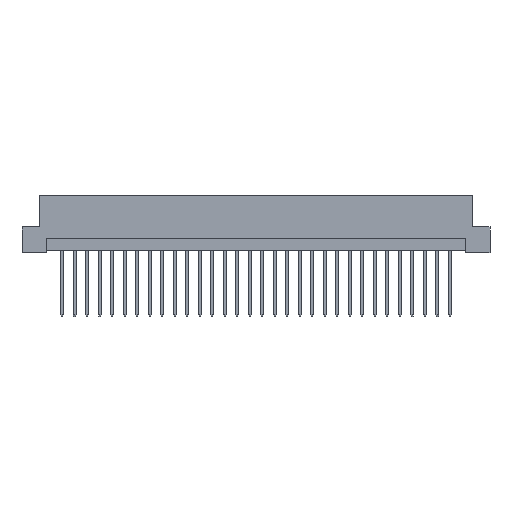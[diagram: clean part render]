
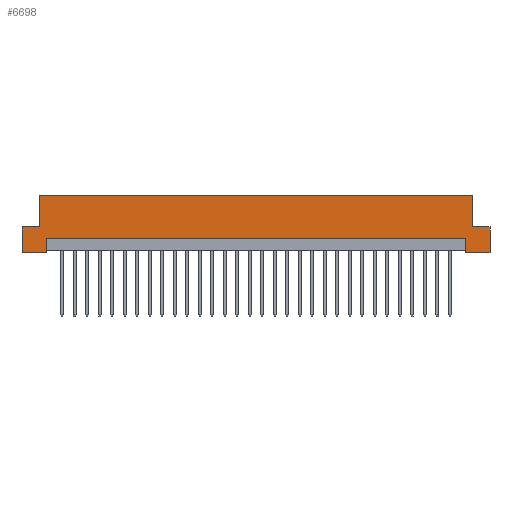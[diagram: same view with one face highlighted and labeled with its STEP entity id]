
A CAD part, front view. The second image highlights one B-rep face of the part: STEP entity #6698.
In plain terms, the highlighted planar face has unit normal (0, -1, 0).
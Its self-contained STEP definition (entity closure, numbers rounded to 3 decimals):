
#183 = VECTOR ( 'NONE', #7089, 1000. ) ;
#334 = DIRECTION ( 'NONE',  ( 1., 0., 0. ) ) ;
#344 = CARTESIAN_POINT ( 'NONE',  ( 44., 0., 11.6 ) ) ;
#518 = CARTESIAN_POINT ( 'NONE',  ( -42.6, 0., 0. ) ) ;
#773 = EDGE_CURVE ( 'NONE', #15670, #1671, #16305, .T. ) ;
#828 = LINE ( 'NONE', #3262, #14759 ) ;
#1134 = LINE ( 'NONE', #2794, #183 ) ;
#1329 = VERTEX_POINT ( 'NONE', #9438 ) ;
#1596 = VERTEX_POINT ( 'NONE', #9137 ) ;
#1671 = VERTEX_POINT ( 'NONE', #344 ) ;
#1858 = CARTESIAN_POINT ( 'NONE',  ( -42.6, 0., 0.5 ) ) ;
#1908 = VECTOR ( 'NONE', #10452, 1000. ) ;
#2086 = VERTEX_POINT ( 'NONE', #518 ) ;
#2103 = EDGE_CURVE ( 'NONE', #15670, #17255, #6191, .T. ) ;
#2208 = LINE ( 'NONE', #7899, #12714 ) ;
#2485 = VECTOR ( 'NONE', #11532, 1000. ) ;
#2656 = VECTOR ( 'NONE', #16609, 1000. ) ;
#2723 = DIRECTION ( 'NONE',  ( 0., 0., 1. ) ) ;
#2794 = CARTESIAN_POINT ( 'NONE',  ( 42.6, 0., 2.9 ) ) ;
#3262 = CARTESIAN_POINT ( 'NONE',  ( 47.5, 0., 0. ) ) ;
#3556 = VECTOR ( 'NONE', #7881, 1000. ) ;
#3605 = CARTESIAN_POINT ( 'NONE',  ( 42.6, 0., 0. ) ) ;
#3652 = VERTEX_POINT ( 'NONE', #17340 ) ;
#3809 = AXIS2_PLACEMENT_3D ( 'NONE', #18094, #5425, #2723 ) ;
#4188 = VECTOR ( 'NONE', #16476, 1000. ) ;
#4403 = CARTESIAN_POINT ( 'NONE',  ( 47.5, 0., 0. ) ) ;
#4410 = EDGE_CURVE ( 'NONE', #2086, #11112, #16179, .T. ) ;
#4904 = VERTEX_POINT ( 'NONE', #4403 ) ;
#4984 = LINE ( 'NONE', #10686, #2656 ) ;
#5258 = CARTESIAN_POINT ( 'NONE',  ( -47.5, 0., 11.6 ) ) ;
#5264 = VERTEX_POINT ( 'NONE', #6732 ) ;
#5296 = ORIENTED_EDGE ( 'NONE', *, *, #12866, .F. ) ;
#5404 = ORIENTED_EDGE ( 'NONE', *, *, #8252, .F. ) ;
#5425 = DIRECTION ( 'NONE',  ( 0., 1., 0. ) ) ;
#5496 = EDGE_CURVE ( 'NONE', #7389, #3652, #1134, .T. ) ;
#6138 = EDGE_CURVE ( 'NONE', #11112, #1329, #7243, .T. ) ;
#6145 = DIRECTION ( 'NONE',  ( 0., 0., -1. ) ) ;
#6191 = LINE ( 'NONE', #9006, #2485 ) ;
#6284 = LINE ( 'NONE', #12209, #3556 ) ;
#6523 = VECTOR ( 'NONE', #7028, 1000. ) ;
#6698 = ADVANCED_FACE ( 'NONE', ( #6839 ), #15374, .F. ) ;
#6732 = CARTESIAN_POINT ( 'NONE',  ( -44., 0., 5.2 ) ) ;
#6839 = FACE_OUTER_BOUND ( 'NONE', #14641, .T. ) ;
#7028 = DIRECTION ( 'NONE',  ( 1., 0., 0. ) ) ;
#7089 = DIRECTION ( 'NONE',  ( -1., 0., 0. ) ) ;
#7243 = LINE ( 'NONE', #7522, #8244 ) ;
#7389 = VERTEX_POINT ( 'NONE', #17563 ) ;
#7522 = CARTESIAN_POINT ( 'NONE',  ( -47.5, 0., 0. ) ) ;
#7668 = CARTESIAN_POINT ( 'NONE',  ( 44., 0., 5.2 ) ) ;
#7676 = CARTESIAN_POINT ( 'NONE',  ( 44., 0., 5.2 ) ) ;
#7881 = DIRECTION ( 'NONE',  ( -1., 0., 0. ) ) ;
#7899 = CARTESIAN_POINT ( 'NONE',  ( -47.5, 0., 5.2 ) ) ;
#8040 = EDGE_CURVE ( 'NONE', #5264, #1596, #4984, .T. ) ;
#8102 = EDGE_CURVE ( 'NONE', #4904, #17877, #6284, .T. ) ;
#8152 = ORIENTED_EDGE ( 'NONE', *, *, #773, .T. ) ;
#8244 = VECTOR ( 'NONE', #17181, 1000. ) ;
#8252 = EDGE_CURVE ( 'NONE', #1596, #1671, #12659, .T. ) ;
#9006 = CARTESIAN_POINT ( 'NONE',  ( 47.5, 0., 5.2 ) ) ;
#9137 = CARTESIAN_POINT ( 'NONE',  ( -44., 0., 11.6 ) ) ;
#9176 = LINE ( 'NONE', #10473, #4188 ) ;
#9438 = CARTESIAN_POINT ( 'NONE',  ( -47.5, 0., 5.2 ) ) ;
#9624 = VECTOR ( 'NONE', #13401, 1000. ) ;
#9909 = ORIENTED_EDGE ( 'NONE', *, *, #4410, .F. ) ;
#9989 = CARTESIAN_POINT ( 'NONE',  ( 47.5, 0., 5.2 ) ) ;
#10452 = DIRECTION ( 'NONE',  ( 0., 0., -1. ) ) ;
#10473 = CARTESIAN_POINT ( 'NONE',  ( 42.6, 0., 0.5 ) ) ;
#10634 = LINE ( 'NONE', #1858, #1908 ) ;
#10686 = CARTESIAN_POINT ( 'NONE',  ( -44., 0., 5.2 ) ) ;
#10796 = ORIENTED_EDGE ( 'NONE', *, *, #6138, .F. ) ;
#11112 = VERTEX_POINT ( 'NONE', #15797 ) ;
#11532 = DIRECTION ( 'NONE',  ( 1., 0., 0. ) ) ;
#12194 = ORIENTED_EDGE ( 'NONE', *, *, #2103, .F. ) ;
#12209 = CARTESIAN_POINT ( 'NONE',  ( -47.5, 0., 0. ) ) ;
#12659 = LINE ( 'NONE', #5258, #6523 ) ;
#12714 = VECTOR ( 'NONE', #334, 1000. ) ;
#12866 = EDGE_CURVE ( 'NONE', #17255, #4904, #828, .T. ) ;
#12905 = EDGE_CURVE ( 'NONE', #3652, #2086, #10634, .T. ) ;
#13170 = ORIENTED_EDGE ( 'NONE', *, *, #13404, .F. ) ;
#13401 = DIRECTION ( 'NONE',  ( 0., 0., 1. ) ) ;
#13404 = EDGE_CURVE ( 'NONE', #1329, #5264, #2208, .T. ) ;
#13725 = ORIENTED_EDGE ( 'NONE', *, *, #5496, .F. ) ;
#14641 = EDGE_LOOP ( 'NONE', ( #13725, #15225, #14972, #5296, #12194, #8152, #5404, #15381, #13170, #10796, #9909, #18252 ) ) ;
#14759 = VECTOR ( 'NONE', #6145, 1000. ) ;
#14972 = ORIENTED_EDGE ( 'NONE', *, *, #8102, .F. ) ;
#15225 = ORIENTED_EDGE ( 'NONE', *, *, #16911, .T. ) ;
#15374 = PLANE ( 'NONE',  #3809 ) ;
#15381 = ORIENTED_EDGE ( 'NONE', *, *, #8040, .F. ) ;
#15670 = VERTEX_POINT ( 'NONE', #7668 ) ;
#15797 = CARTESIAN_POINT ( 'NONE',  ( -47.5, 0., 0. ) ) ;
#16091 = DIRECTION ( 'NONE',  ( -1., 0., 0. ) ) ;
#16179 = LINE ( 'NONE', #17486, #16878 ) ;
#16305 = LINE ( 'NONE', #7676, #9624 ) ;
#16476 = DIRECTION ( 'NONE',  ( 0., 0., -1. ) ) ;
#16609 = DIRECTION ( 'NONE',  ( 0., 0., 1. ) ) ;
#16878 = VECTOR ( 'NONE', #16091, 1000. ) ;
#16911 = EDGE_CURVE ( 'NONE', #7389, #17877, #9176, .T. ) ;
#17181 = DIRECTION ( 'NONE',  ( 0., 0., 1. ) ) ;
#17255 = VERTEX_POINT ( 'NONE', #9989 ) ;
#17340 = CARTESIAN_POINT ( 'NONE',  ( -42.6, 0., 2.9 ) ) ;
#17486 = CARTESIAN_POINT ( 'NONE',  ( -47.5, 0., 0. ) ) ;
#17563 = CARTESIAN_POINT ( 'NONE',  ( 42.6, 0., 2.9 ) ) ;
#17877 = VERTEX_POINT ( 'NONE', #3605 ) ;
#18094 = CARTESIAN_POINT ( 'NONE',  ( -47.5, 0., 11.6 ) ) ;
#18252 = ORIENTED_EDGE ( 'NONE', *, *, #12905, .F. ) ;
